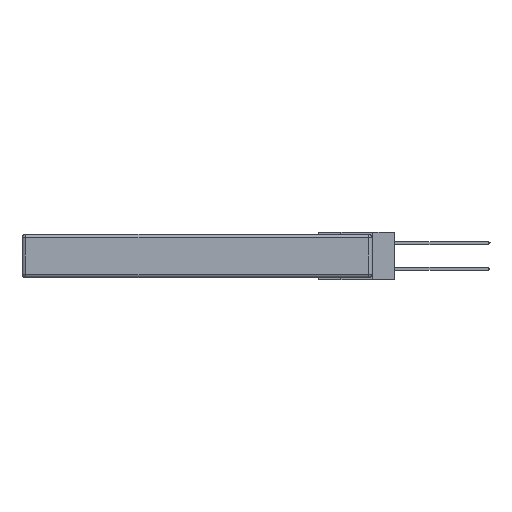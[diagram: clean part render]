
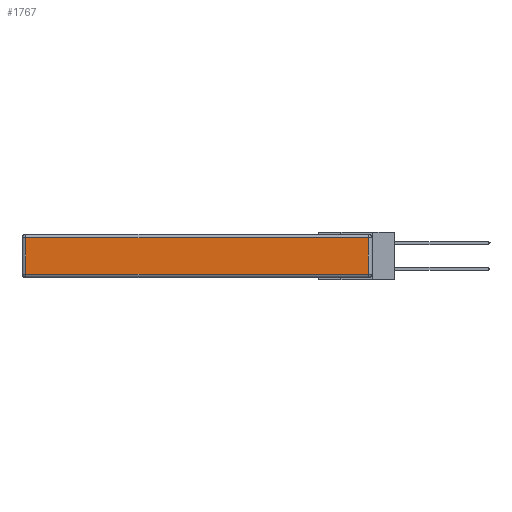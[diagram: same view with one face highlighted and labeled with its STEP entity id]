
A CAD part, left-side view. The second image highlights one B-rep face of the part: STEP entity #1767.
In plain terms, the highlighted planar face has unit normal (-1, 0, 0).
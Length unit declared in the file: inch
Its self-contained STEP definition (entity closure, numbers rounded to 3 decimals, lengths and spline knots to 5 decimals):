
#32 = LINE ( 'NONE', #8733, #31196 ) ;
#1767 = ADVANCED_FACE ( 'NONE', ( #32337 ), #27634, .T. ) ;
#1888 = VERTEX_POINT ( 'NONE', #21012 ) ;
#3956 = CARTESIAN_POINT ( 'NONE',  ( 0., 0., -0.343 ) ) ;
#6630 = CARTESIAN_POINT ( 'NONE',  ( 0., 2.72, -0.343 ) ) ;
#8733 = CARTESIAN_POINT ( 'NONE',  ( 0., 2.75, -0.03 ) ) ;
#8996 = VERTEX_POINT ( 'NONE', #14503 ) ;
#9499 = VERTEX_POINT ( 'NONE', #16917 ) ;
#10004 = CARTESIAN_POINT ( 'NONE',  ( 0., 0., -0.313 ) ) ;
#12909 = EDGE_CURVE ( 'NONE', #32700, #1888, #24202, .T. ) ;
#14260 = DIRECTION ( 'NONE',  ( 0., 0., 1. ) ) ;
#14503 = CARTESIAN_POINT ( 'NONE',  ( 0., 0.03, -0.313 ) ) ;
#14505 = VECTOR ( 'NONE', #28384, 39.37008 ) ;
#14703 = DIRECTION ( 'NONE',  ( -1., 0., 0. ) ) ;
#16202 = DIRECTION ( 'NONE',  ( 0., 1., 0. ) ) ;
#16379 = ORIENTED_EDGE ( 'NONE', *, *, #23100, .T. ) ;
#16726 = EDGE_LOOP ( 'NONE', ( #33011, #26768, #16379, #21497 ) ) ;
#16917 = CARTESIAN_POINT ( 'NONE',  ( 0., 0.03, -0.03 ) ) ;
#17067 = DIRECTION ( 'NONE',  ( 0., 0., 1. ) ) ;
#17503 = CARTESIAN_POINT ( 'NONE',  ( 0., 2.72, -0.03 ) ) ;
#19436 = DIRECTION ( 'NONE',  ( 0., 0., -1. ) ) ;
#21012 = CARTESIAN_POINT ( 'NONE',  ( 0., 2.72, -0.313 ) ) ;
#21497 = ORIENTED_EDGE ( 'NONE', *, *, #12909, .T. ) ;
#21909 = EDGE_CURVE ( 'NONE', #8996, #9499, #28030, .T. ) ;
#22187 = CARTESIAN_POINT ( 'NONE',  ( 0., 0.03, -0.343 ) ) ;
#23100 = EDGE_CURVE ( 'NONE', #9499, #32700, #32, .T. ) ;
#24202 = LINE ( 'NONE', #6630, #27500 ) ;
#24437 = EDGE_CURVE ( 'NONE', #1888, #8996, #30750, .T. ) ;
#26768 = ORIENTED_EDGE ( 'NONE', *, *, #21909, .T. ) ;
#27109 = AXIS2_PLACEMENT_3D ( 'NONE', #3956, #14703, #14260 ) ;
#27500 = VECTOR ( 'NONE', #19436, 39.37008 ) ;
#27634 = PLANE ( 'NONE',  #27109 ) ;
#28030 = LINE ( 'NONE', #22187, #32478 ) ;
#28384 = DIRECTION ( 'NONE',  ( 0., -1., 0. ) ) ;
#30750 = LINE ( 'NONE', #10004, #14505 ) ;
#31196 = VECTOR ( 'NONE', #16202, 39.37008 ) ;
#32337 = FACE_OUTER_BOUND ( 'NONE', #16726, .T. ) ;
#32478 = VECTOR ( 'NONE', #17067, 39.37008 ) ;
#32700 = VERTEX_POINT ( 'NONE', #17503 ) ;
#33011 = ORIENTED_EDGE ( 'NONE', *, *, #24437, .T. ) ;
